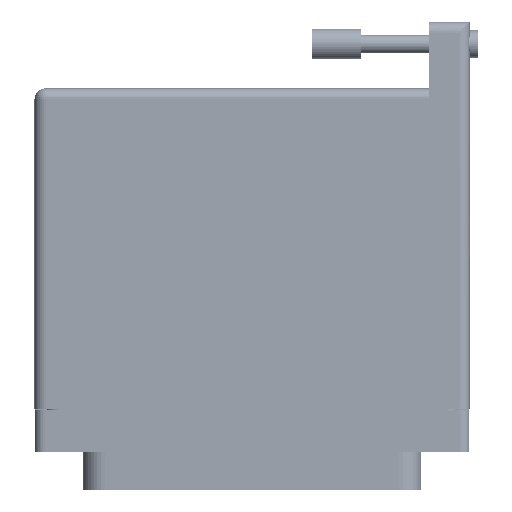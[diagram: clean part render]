
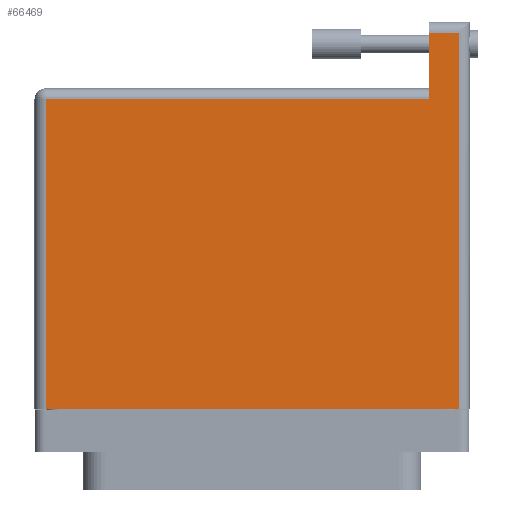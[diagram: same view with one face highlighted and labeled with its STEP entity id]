
A CAD part, front view. The second image highlights one B-rep face of the part: STEP entity #66469.
In plain terms, the highlighted face is planar.
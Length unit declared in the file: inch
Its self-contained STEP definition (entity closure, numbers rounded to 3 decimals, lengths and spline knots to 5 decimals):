
#760 = LINE ( 'NONE', #48870, #65617 ) ;
#1193 = VERTEX_POINT ( 'NONE', #53084 ) ;
#4759 = VECTOR ( 'NONE', #12746, 39.37008 ) ;
#5467 = VERTEX_POINT ( 'NONE', #31899 ) ;
#5562 = CARTESIAN_POINT ( 'NONE',  ( -1.3075, -0.1, 0.765 ) ) ;
#5810 = DIRECTION ( 'NONE',  ( 0., 0., -1. ) ) ;
#7023 = CARTESIAN_POINT ( 'NONE',  ( -1.3775, 1.86, 0.765 ) ) ;
#7566 = CARTESIAN_POINT ( 'NONE',  ( -1.3775, -0.1, 0.765 ) ) ;
#8384 = VECTOR ( 'NONE', #51382, 39.37008 ) ;
#9187 = LINE ( 'NONE', #5562, #4759 ) ;
#11812 = VECTOR ( 'NONE', #80175, 39.37008 ) ;
#12430 = EDGE_LOOP ( 'NONE', ( #22483, #43708, #64679, #12489, #27488, #76712 ) ) ;
#12489 = ORIENTED_EDGE ( 'NONE', *, *, #19627, .T. ) ;
#12746 = DIRECTION ( 'NONE',  ( 0., -1., 0. ) ) ;
#13587 = EDGE_CURVE ( 'NONE', #21719, #19097, #59410, .T. ) ;
#15224 = CARTESIAN_POINT ( 'NONE',  ( 1.3075, -0.1, 0.765 ) ) ;
#19078 = EDGE_CURVE ( 'NONE', #5467, #84258, #9187, .T. ) ;
#19097 = VERTEX_POINT ( 'NONE', #27787 ) ;
#19445 = DIRECTION ( 'NONE',  ( 0., 1., 0. ) ) ;
#19627 = EDGE_CURVE ( 'NONE', #84258, #45141, #62176, .T. ) ;
#21719 = VERTEX_POINT ( 'NONE', #76297 ) ;
#22483 = ORIENTED_EDGE ( 'NONE', *, *, #13587, .T. ) ;
#27488 = ORIENTED_EDGE ( 'NONE', *, *, #71291, .T. ) ;
#27787 = CARTESIAN_POINT ( 'NONE',  ( 1.1215, 1.86, 0.765 ) ) ;
#28034 = CARTESIAN_POINT ( 'NONE',  ( -1.3775, 1.93, 0.765 ) ) ;
#29931 = CARTESIAN_POINT ( 'NONE',  ( -1.3775, 2.28, 0.765 ) ) ;
#31899 = CARTESIAN_POINT ( 'NONE',  ( -1.3075, 1.86, 0.765 ) ) ;
#35956 = VECTOR ( 'NONE', #90705, 39.37008 ) ;
#37471 = AXIS2_PLACEMENT_3D ( 'NONE', #28034, #5810, #41806 ) ;
#40534 = VECTOR ( 'NONE', #65852, 39.37008 ) ;
#41636 = CARTESIAN_POINT ( 'NONE',  ( 1.1215, 2.35, 0.765 ) ) ;
#41806 = DIRECTION ( 'NONE',  ( -1., 0., 0. ) ) ;
#43708 = ORIENTED_EDGE ( 'NONE', *, *, #57686, .T. ) ;
#44015 = FACE_OUTER_BOUND ( 'NONE', #12430, .T. ) ;
#45141 = VERTEX_POINT ( 'NONE', #15224 ) ;
#48870 = CARTESIAN_POINT ( 'NONE',  ( 1.3075, 2.35, 0.765 ) ) ;
#51382 = DIRECTION ( 'NONE',  ( 1., 0., 0. ) ) ;
#53084 = CARTESIAN_POINT ( 'NONE',  ( 1.3075, 2.28, 0.765 ) ) ;
#57686 = EDGE_CURVE ( 'NONE', #19097, #5467, #80110, .T. ) ;
#59410 = LINE ( 'NONE', #41636, #35956 ) ;
#62176 = LINE ( 'NONE', #7566, #8384 ) ;
#64679 = ORIENTED_EDGE ( 'NONE', *, *, #19078, .T. ) ;
#65617 = VECTOR ( 'NONE', #19445, 39.37008 ) ;
#65852 = DIRECTION ( 'NONE',  ( -1., 0., 0. ) ) ;
#66469 = ADVANCED_FACE ( 'NONE', ( #44015 ), #70829, .F. ) ;
#67294 = EDGE_CURVE ( 'NONE', #1193, #21719, #69592, .T. ) ;
#69592 = LINE ( 'NONE', #29931, #40534 ) ;
#70829 = PLANE ( 'NONE',  #37471 ) ;
#71291 = EDGE_CURVE ( 'NONE', #45141, #1193, #760, .T. ) ;
#76297 = CARTESIAN_POINT ( 'NONE',  ( 1.1215, 2.28, 0.765 ) ) ;
#76712 = ORIENTED_EDGE ( 'NONE', *, *, #67294, .T. ) ;
#80110 = LINE ( 'NONE', #7023, #11812 ) ;
#80175 = DIRECTION ( 'NONE',  ( -1., 0., 0. ) ) ;
#84258 = VERTEX_POINT ( 'NONE', #92006 ) ;
#90705 = DIRECTION ( 'NONE',  ( 0., -1., 0. ) ) ;
#92006 = CARTESIAN_POINT ( 'NONE',  ( -1.3075, -0.1, 0.765 ) ) ;
